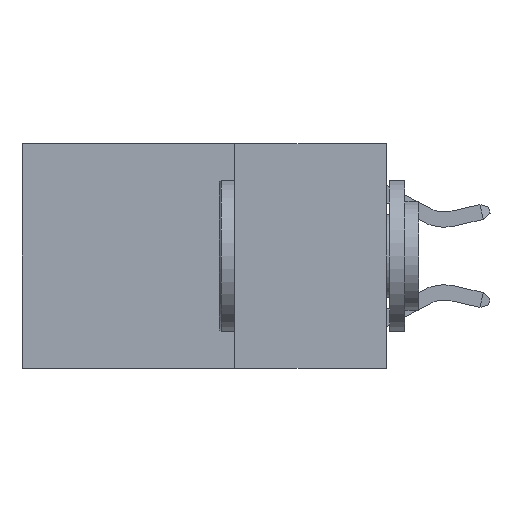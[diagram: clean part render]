
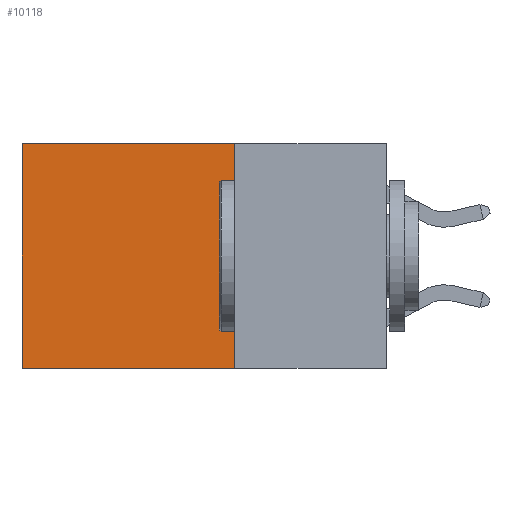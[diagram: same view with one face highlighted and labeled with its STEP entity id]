
A CAD part, left-side view. The second image highlights one B-rep face of the part: STEP entity #10118.
In plain terms, the highlighted planar face has unit normal (-1, 0, 0).
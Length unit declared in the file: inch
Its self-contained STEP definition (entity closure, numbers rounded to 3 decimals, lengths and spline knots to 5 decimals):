
#249 = CARTESIAN_POINT ( 'NONE',  ( 0.2625, 0.25, -0.37 ) ) ;
#372 = VERTEX_POINT ( 'NONE', #1145 ) ;
#751 = CARTESIAN_POINT ( 'NONE',  ( 0.2625, 0.6, -0.37 ) ) ;
#764 = VECTOR ( 'NONE', #6108, 39.37008 ) ;
#1145 = CARTESIAN_POINT ( 'NONE',  ( 0.2625, 0.25, 0. ) ) ;
#1276 = VECTOR ( 'NONE', #2807, 39.37008 ) ;
#2221 = CARTESIAN_POINT ( 'NONE',  ( 0.2625, 0.25, 0. ) ) ;
#2807 = DIRECTION ( 'NONE',  ( 0., 1., 0. ) ) ;
#3057 = ORIENTED_EDGE ( 'NONE', *, *, #8379, .F. ) ;
#3202 = EDGE_CURVE ( 'NONE', #14501, #5969, #12680, .T. ) ;
#3447 = FACE_OUTER_BOUND ( 'NONE', #10536, .T. ) ;
#4376 = LINE ( 'NONE', #6155, #1276 ) ;
#4595 = LINE ( 'NONE', #11929, #764 ) ;
#5548 = DIRECTION ( 'NONE',  ( 1., 0., 0. ) ) ;
#5969 = VERTEX_POINT ( 'NONE', #751 ) ;
#5970 = AXIS2_PLACEMENT_3D ( 'NONE', #10015, #5548, #13660 ) ;
#6108 = DIRECTION ( 'NONE',  ( 0., 1., 0. ) ) ;
#6155 = CARTESIAN_POINT ( 'NONE',  ( 0.2625, 0.25, 0. ) ) ;
#6757 = DIRECTION ( 'NONE',  ( 0., 0., -1. ) ) ;
#7383 = EDGE_CURVE ( 'NONE', #372, #14761, #11031, .T. ) ;
#7613 = VECTOR ( 'NONE', #6757, 39.37008 ) ;
#8379 = EDGE_CURVE ( 'NONE', #14761, #5969, #4595, .T. ) ;
#8693 = ORIENTED_EDGE ( 'NONE', *, *, #3202, .T. ) ;
#9038 = CARTESIAN_POINT ( 'NONE',  ( 0.2625, 0.6, 0. ) ) ;
#9102 = VECTOR ( 'NONE', #10683, 39.37008 ) ;
#9197 = ORIENTED_EDGE ( 'NONE', *, *, #10467, .T. ) ;
#10015 = CARTESIAN_POINT ( 'NONE',  ( 0.2625, 0.25, 0. ) ) ;
#10118 = ADVANCED_FACE ( 'NONE', ( #3447 ), #12514, .F. ) ;
#10467 = EDGE_CURVE ( 'NONE', #372, #14501, #4376, .T. ) ;
#10536 = EDGE_LOOP ( 'NONE', ( #8693, #3057, #10879, #9197 ) ) ;
#10683 = DIRECTION ( 'NONE',  ( 0., 0., -1. ) ) ;
#10879 = ORIENTED_EDGE ( 'NONE', *, *, #7383, .F. ) ;
#11031 = LINE ( 'NONE', #2221, #7613 ) ;
#11929 = CARTESIAN_POINT ( 'NONE',  ( 0.2625, 0.25, -0.37 ) ) ;
#12514 = PLANE ( 'NONE',  #5970 ) ;
#12680 = LINE ( 'NONE', #13087, #9102 ) ;
#13087 = CARTESIAN_POINT ( 'NONE',  ( 0.2625, 0.6, 0. ) ) ;
#13660 = DIRECTION ( 'NONE',  ( 0., 0., -1. ) ) ;
#14501 = VERTEX_POINT ( 'NONE', #9038 ) ;
#14761 = VERTEX_POINT ( 'NONE', #249 ) ;
